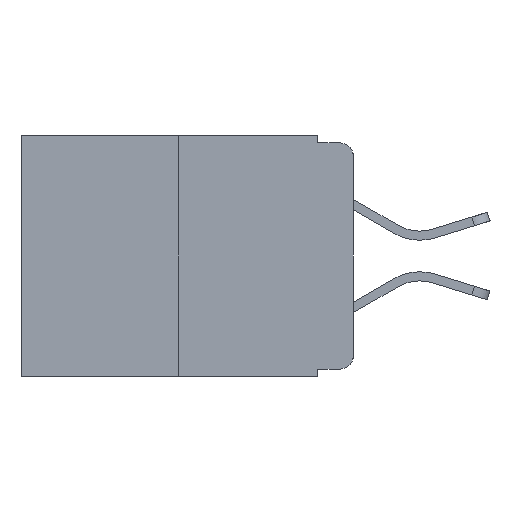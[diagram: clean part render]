
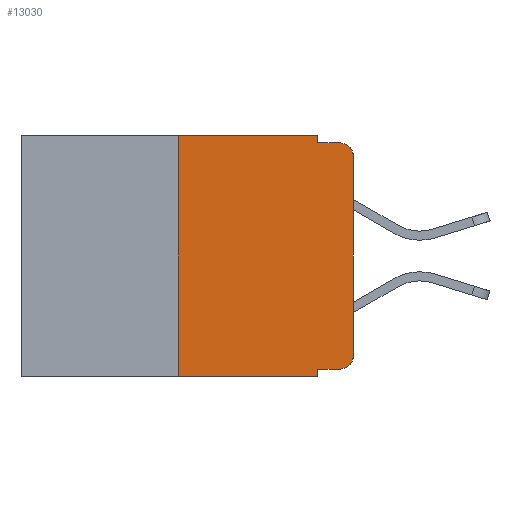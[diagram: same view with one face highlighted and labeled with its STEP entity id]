
A CAD part, left-side view. The second image highlights one B-rep face of the part: STEP entity #13030.
In plain terms, the highlighted planar face has unit normal (-1, 0, 0).
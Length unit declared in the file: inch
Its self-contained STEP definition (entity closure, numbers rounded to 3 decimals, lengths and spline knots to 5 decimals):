
#50 = CARTESIAN_POINT ( 'NONE',  ( 0., 0.051, -0.01 ) ) ;
#238 = CARTESIAN_POINT ( 'NONE',  ( 0., 0.02, -0.03 ) ) ;
#570 = CARTESIAN_POINT ( 'NONE',  ( 0., 0.02, -0.333 ) ) ;
#597 = DIRECTION ( 'NONE',  ( 0., 0., 1. ) ) ;
#759 = EDGE_CURVE ( 'NONE', #8766, #879, #11755, .T. ) ;
#879 = VERTEX_POINT ( 'NONE', #3579 ) ;
#1204 = VECTOR ( 'NONE', #6131, 39.37008 ) ;
#1729 = EDGE_CURVE ( 'NONE', #879, #10656, #11706, .T. ) ;
#2012 = VECTOR ( 'NONE', #7080, 39.37008 ) ;
#2143 = CARTESIAN_POINT ( 'NONE',  ( 0., 0.051, 0. ) ) ;
#2280 = VECTOR ( 'NONE', #10999, 39.37008 ) ;
#2304 = DIRECTION ( 'NONE',  ( 0., 0., -1. ) ) ;
#2450 = DIRECTION ( 'NONE',  ( -1., 0., 0. ) ) ;
#2583 = VERTEX_POINT ( 'NONE', #6690 ) ;
#2584 = EDGE_CURVE ( 'NONE', #12536, #8766, #15405, .T. ) ;
#2880 = AXIS2_PLACEMENT_3D ( 'NONE', #11393, #4255, #12578 ) ;
#2929 = CARTESIAN_POINT ( 'NONE',  ( 0., 0.051, -0.333 ) ) ;
#3173 = CARTESIAN_POINT ( 'NONE',  ( 0., 0.02, -0.313 ) ) ;
#3206 = FACE_OUTER_BOUND ( 'NONE', #3754, .T. ) ;
#3579 = CARTESIAN_POINT ( 'NONE',  ( 0., 0., -0.03 ) ) ;
#3754 = EDGE_LOOP ( 'NONE', ( #8044, #11565, #9158, #12315, #12658, #13022, #7116, #13380, #13721, #5057 ) ) ;
#4021 = LINE ( 'NONE', #2929, #13115 ) ;
#4202 = EDGE_CURVE ( 'NONE', #8116, #12536, #4021, .T. ) ;
#4245 = EDGE_CURVE ( 'NONE', #9875, #2583, #12751, .T. ) ;
#4255 = DIRECTION ( 'NONE',  ( 1., 0., 0. ) ) ;
#4310 = CARTESIAN_POINT ( 'NONE',  ( 0., 0.25, 0. ) ) ;
#5057 = ORIENTED_EDGE ( 'NONE', *, *, #2584, .T. ) ;
#5318 = EDGE_CURVE ( 'NONE', #9875, #7163, #10875, .T. ) ;
#5432 = PLANE ( 'NONE',  #2880 ) ;
#5446 = VECTOR ( 'NONE', #597, 39.37008 ) ;
#5501 = CARTESIAN_POINT ( 'NONE',  ( 0., 0.051, 0. ) ) ;
#5577 = CARTESIAN_POINT ( 'NONE',  ( 0., 0.02, -0.01 ) ) ;
#5705 = DIRECTION ( 'NONE',  ( 0., -1., 0. ) ) ;
#6131 = DIRECTION ( 'NONE',  ( 0., 0., 1. ) ) ;
#6304 = VECTOR ( 'NONE', #14297, 39.37008 ) ;
#6377 = CARTESIAN_POINT ( 'NONE',  ( 0., 0.25, -0.343 ) ) ;
#6381 = DIRECTION ( 'NONE',  ( 0., -1., 0. ) ) ;
#6423 = CARTESIAN_POINT ( 'NONE',  ( 0., 0.25, 0. ) ) ;
#6690 = CARTESIAN_POINT ( 'NONE',  ( 0., 0.051, -0.343 ) ) ;
#6897 = VECTOR ( 'NONE', #9299, 39.37008 ) ;
#7080 = DIRECTION ( 'NONE',  ( 0., -1., 0. ) ) ;
#7116 = ORIENTED_EDGE ( 'NONE', *, *, #4245, .T. ) ;
#7128 = EDGE_CURVE ( 'NONE', #12246, #10656, #14598, .T. ) ;
#7163 = VERTEX_POINT ( 'NONE', #4310 ) ;
#8044 = ORIENTED_EDGE ( 'NONE', *, *, #759, .T. ) ;
#8116 = VERTEX_POINT ( 'NONE', #8828 ) ;
#8766 = VERTEX_POINT ( 'NONE', #15500 ) ;
#8793 = AXIS2_PLACEMENT_3D ( 'NONE', #3173, #2450, #2304 ) ;
#8828 = CARTESIAN_POINT ( 'NONE',  ( 0., 0.051, -0.333 ) ) ;
#9021 = EDGE_CURVE ( 'NONE', #15598, #12246, #13503, .T. ) ;
#9158 = ORIENTED_EDGE ( 'NONE', *, *, #7128, .F. ) ;
#9244 = VECTOR ( 'NONE', #6381, 39.37008 ) ;
#9297 = EDGE_CURVE ( 'NONE', #8116, #2583, #9464, .T. ) ;
#9299 = DIRECTION ( 'NONE',  ( 0., 0., -1. ) ) ;
#9464 = LINE ( 'NONE', #2143, #6304 ) ;
#9825 = CARTESIAN_POINT ( 'NONE',  ( 0., 0.473, 0. ) ) ;
#9852 = CARTESIAN_POINT ( 'NONE',  ( 0., 0.051, -0.01 ) ) ;
#9875 = VERTEX_POINT ( 'NONE', #6377 ) ;
#10607 = DIRECTION ( 'NONE',  ( -1., 0., 0. ) ) ;
#10645 = DIRECTION ( 'NONE',  ( 0., 0., -1. ) ) ;
#10656 = VERTEX_POINT ( 'NONE', #5577 ) ;
#10742 = AXIS2_PLACEMENT_3D ( 'NONE', #238, #10607, #10645 ) ;
#10875 = LINE ( 'NONE', #6423, #1204 ) ;
#10999 = DIRECTION ( 'NONE',  ( 0., -1., 0. ) ) ;
#11393 = CARTESIAN_POINT ( 'NONE',  ( 0., 0.473, 0. ) ) ;
#11528 = EDGE_CURVE ( 'NONE', #7163, #15598, #11827, .T. ) ;
#11565 = ORIENTED_EDGE ( 'NONE', *, *, #1729, .T. ) ;
#11706 = CIRCLE ( 'NONE', #10742, 0.02 ) ;
#11755 = LINE ( 'NONE', #13976, #5446 ) ;
#11827 = LINE ( 'NONE', #9825, #2280 ) ;
#12246 = VERTEX_POINT ( 'NONE', #9852 ) ;
#12315 = ORIENTED_EDGE ( 'NONE', *, *, #9021, .F. ) ;
#12446 = CARTESIAN_POINT ( 'NONE',  ( 0., 0.473, -0.343 ) ) ;
#12536 = VERTEX_POINT ( 'NONE', #570 ) ;
#12578 = DIRECTION ( 'NONE',  ( 0., 0., -1. ) ) ;
#12658 = ORIENTED_EDGE ( 'NONE', *, *, #11528, .F. ) ;
#12751 = LINE ( 'NONE', #12446, #9244 ) ;
#13022 = ORIENTED_EDGE ( 'NONE', *, *, #5318, .F. ) ;
#13030 = ADVANCED_FACE ( 'NONE', ( #3206 ), #5432, .F. ) ;
#13115 = VECTOR ( 'NONE', #5705, 39.37008 ) ;
#13380 = ORIENTED_EDGE ( 'NONE', *, *, #9297, .F. ) ;
#13503 = LINE ( 'NONE', #15063, #6897 ) ;
#13721 = ORIENTED_EDGE ( 'NONE', *, *, #4202, .T. ) ;
#13976 = CARTESIAN_POINT ( 'NONE',  ( 0., 0., 0. ) ) ;
#14297 = DIRECTION ( 'NONE',  ( 0., 0., -1. ) ) ;
#14598 = LINE ( 'NONE', #50, #2012 ) ;
#15063 = CARTESIAN_POINT ( 'NONE',  ( 0., 0.051, 0. ) ) ;
#15405 = CIRCLE ( 'NONE', #8793, 0.02 ) ;
#15500 = CARTESIAN_POINT ( 'NONE',  ( 0., 0., -0.313 ) ) ;
#15598 = VERTEX_POINT ( 'NONE', #5501 ) ;
